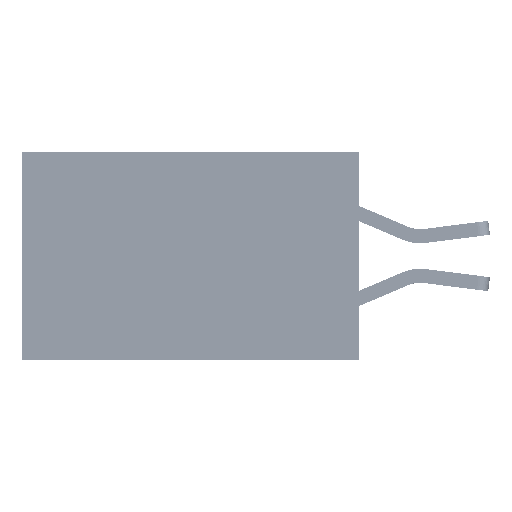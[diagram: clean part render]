
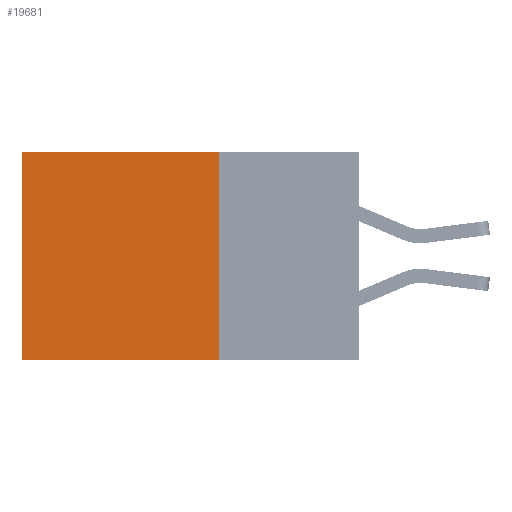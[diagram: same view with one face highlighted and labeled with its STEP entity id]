
A CAD part, left-side view. The second image highlights one B-rep face of the part: STEP entity #19681.
In plain terms, the highlighted planar face has unit normal (-1, 0, 0).
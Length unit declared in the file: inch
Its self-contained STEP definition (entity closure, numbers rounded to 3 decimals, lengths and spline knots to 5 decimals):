
#622 = EDGE_CURVE ( 'NONE', #7232, #28775, #15592, .T. ) ;
#5009 = CARTESIAN_POINT ( 'NONE',  ( 0.2875, 0.25, 0. ) ) ;
#5900 = LINE ( 'NONE', #26506, #21770 ) ;
#7144 = LINE ( 'NONE', #17588, #25258 ) ;
#7232 = VERTEX_POINT ( 'NONE', #5009 ) ;
#8225 = DIRECTION ( 'NONE',  ( 0., 1., 0. ) ) ;
#8824 = DIRECTION ( 'NONE',  ( 0., 0., -1. ) ) ;
#9560 = DIRECTION ( 'NONE',  ( 0., 0., -1. ) ) ;
#10359 = LINE ( 'NONE', #23263, #26873 ) ;
#10408 = ORIENTED_EDGE ( 'NONE', *, *, #38021, .T. ) ;
#10902 = PLANE ( 'NONE',  #17326 ) ;
#11175 = VECTOR ( 'NONE', #8225, 39.37008 ) ;
#13303 = ORIENTED_EDGE ( 'NONE', *, *, #28265, .F. ) ;
#14425 = DIRECTION ( 'NONE',  ( 1., 0., 0. ) ) ;
#15592 = LINE ( 'NONE', #36740, #11175 ) ;
#17097 = EDGE_CURVE ( 'NONE', #32422, #17810, #7144, .T. ) ;
#17326 = AXIS2_PLACEMENT_3D ( 'NONE', #21027, #14425, #45593 ) ;
#17588 = CARTESIAN_POINT ( 'NONE',  ( 0.2875, 0.25, -0.37 ) ) ;
#17810 = VERTEX_POINT ( 'NONE', #28153 ) ;
#19681 = ADVANCED_FACE ( 'NONE', ( #32178 ), #10902, .F. ) ;
#21027 = CARTESIAN_POINT ( 'NONE',  ( 0.2875, 0.25, 0. ) ) ;
#21770 = VECTOR ( 'NONE', #9560, 39.37008 ) ;
#23263 = CARTESIAN_POINT ( 'NONE',  ( 0.2875, 0.25, 0. ) ) ;
#25258 = VECTOR ( 'NONE', #42451, 39.37008 ) ;
#26506 = CARTESIAN_POINT ( 'NONE',  ( 0.2875, 0.6, 0. ) ) ;
#26873 = VECTOR ( 'NONE', #8824, 39.37008 ) ;
#28153 = CARTESIAN_POINT ( 'NONE',  ( 0.2875, 0.6, -0.37 ) ) ;
#28265 = EDGE_CURVE ( 'NONE', #7232, #32422, #10359, .T. ) ;
#28775 = VERTEX_POINT ( 'NONE', #36532 ) ;
#30290 = ORIENTED_EDGE ( 'NONE', *, *, #622, .T. ) ;
#30946 = CARTESIAN_POINT ( 'NONE',  ( 0.2875, 0.25, -0.37 ) ) ;
#32178 = FACE_OUTER_BOUND ( 'NONE', #32805, .T. ) ;
#32422 = VERTEX_POINT ( 'NONE', #30946 ) ;
#32805 = EDGE_LOOP ( 'NONE', ( #10408, #44584, #13303, #30290 ) ) ;
#36532 = CARTESIAN_POINT ( 'NONE',  ( 0.2875, 0.6, 0. ) ) ;
#36740 = CARTESIAN_POINT ( 'NONE',  ( 0.2875, 0.25, 0. ) ) ;
#38021 = EDGE_CURVE ( 'NONE', #28775, #17810, #5900, .T. ) ;
#42451 = DIRECTION ( 'NONE',  ( 0., 1., 0. ) ) ;
#44584 = ORIENTED_EDGE ( 'NONE', *, *, #17097, .F. ) ;
#45593 = DIRECTION ( 'NONE',  ( 0., 0., -1. ) ) ;
